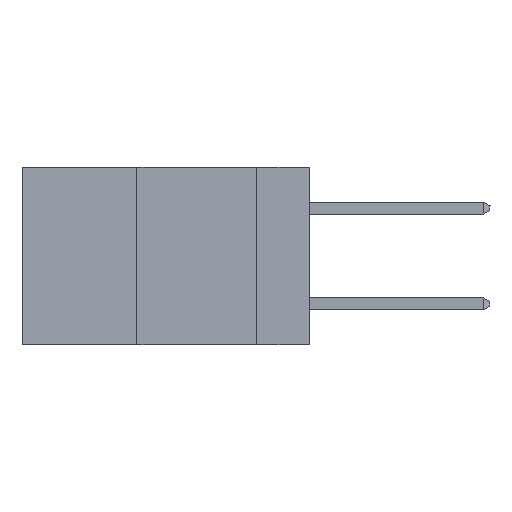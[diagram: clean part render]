
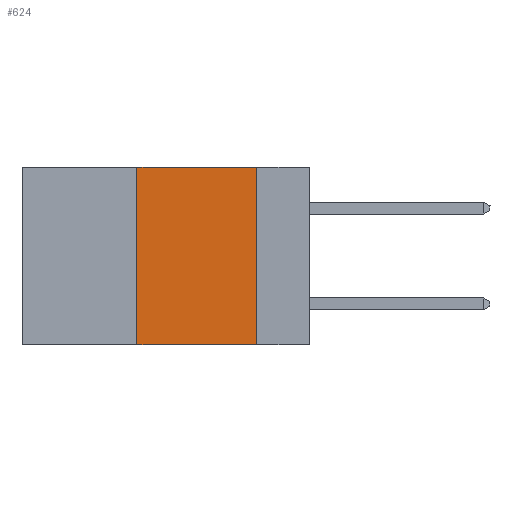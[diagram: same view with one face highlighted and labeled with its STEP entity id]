
A CAD part, left-side view. The second image highlights one B-rep face of the part: STEP entity #624.
In plain terms, the highlighted planar face has unit normal (-1, 0, 0).
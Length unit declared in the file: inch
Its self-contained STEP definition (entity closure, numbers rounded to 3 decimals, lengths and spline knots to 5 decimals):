
#193 = LINE ( 'NONE', #8239, #1046 ) ;
#606 = VECTOR ( 'NONE', #826, 39.37008 ) ;
#624 = ADVANCED_FACE ( 'NONE', ( #1282 ), #722, .F. ) ;
#722 = PLANE ( 'NONE',  #8079 ) ;
#826 = DIRECTION ( 'NONE',  ( 0., 0., 1. ) ) ;
#911 = DIRECTION ( 'NONE',  ( 1., 0., 0. ) ) ;
#924 = CARTESIAN_POINT ( 'NONE',  ( 0., 0.36, 0. ) ) ;
#1040 = CARTESIAN_POINT ( 'NONE',  ( 0., 0.11, -0.37 ) ) ;
#1046 = VECTOR ( 'NONE', #13851, 39.37008 ) ;
#1282 = FACE_OUTER_BOUND ( 'NONE', #2867, .T. ) ;
#1408 = ORIENTED_EDGE ( 'NONE', *, *, #13536, .F. ) ;
#2149 = DIRECTION ( 'NONE',  ( 0., -1., 0. ) ) ;
#2867 = EDGE_LOOP ( 'NONE', ( #1408, #12847, #3475, #13806 ) ) ;
#3350 = DIRECTION ( 'NONE',  ( 0., 0., -1. ) ) ;
#3421 = LINE ( 'NONE', #4496, #5532 ) ;
#3429 = DIRECTION ( 'NONE',  ( 0., 0., -1. ) ) ;
#3475 = ORIENTED_EDGE ( 'NONE', *, *, #11775, .F. ) ;
#3534 = EDGE_CURVE ( 'NONE', #5243, #12985, #193, .T. ) ;
#3832 = LINE ( 'NONE', #924, #606 ) ;
#4134 = CARTESIAN_POINT ( 'NONE',  ( 0., 0.6, 0. ) ) ;
#4496 = CARTESIAN_POINT ( 'NONE',  ( 0., 0.11, 0. ) ) ;
#4564 = EDGE_CURVE ( 'NONE', #13691, #7714, #7689, .T. ) ;
#5243 = VERTEX_POINT ( 'NONE', #13425 ) ;
#5532 = VECTOR ( 'NONE', #3429, 39.37008 ) ;
#7689 = LINE ( 'NONE', #13084, #12833 ) ;
#7714 = VERTEX_POINT ( 'NONE', #1040 ) ;
#8079 = AXIS2_PLACEMENT_3D ( 'NONE', #4134, #911, #3350 ) ;
#8239 = CARTESIAN_POINT ( 'NONE',  ( 0., 0.6, 0. ) ) ;
#11775 = EDGE_CURVE ( 'NONE', #13691, #5243, #3832, .T. ) ;
#12088 = CARTESIAN_POINT ( 'NONE',  ( 0., 0.11, 0. ) ) ;
#12833 = VECTOR ( 'NONE', #2149, 39.37008 ) ;
#12847 = ORIENTED_EDGE ( 'NONE', *, *, #3534, .F. ) ;
#12985 = VERTEX_POINT ( 'NONE', #12088 ) ;
#13084 = CARTESIAN_POINT ( 'NONE',  ( 0., 0.6, -0.37 ) ) ;
#13425 = CARTESIAN_POINT ( 'NONE',  ( 0., 0.36, 0. ) ) ;
#13444 = CARTESIAN_POINT ( 'NONE',  ( 0., 0.36, -0.37 ) ) ;
#13536 = EDGE_CURVE ( 'NONE', #12985, #7714, #3421, .T. ) ;
#13691 = VERTEX_POINT ( 'NONE', #13444 ) ;
#13806 = ORIENTED_EDGE ( 'NONE', *, *, #4564, .T. ) ;
#13851 = DIRECTION ( 'NONE',  ( 0., -1., 0. ) ) ;
